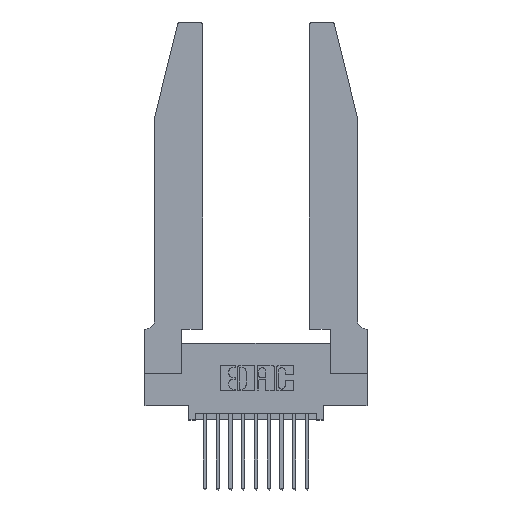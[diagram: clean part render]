
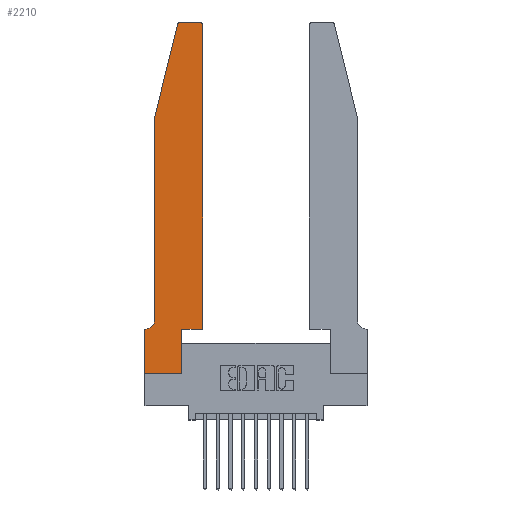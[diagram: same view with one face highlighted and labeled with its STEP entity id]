
A CAD part, top view. The second image highlights one B-rep face of the part: STEP entity #2210.
In plain terms, the highlighted planar face has unit normal (0, 0, 1).
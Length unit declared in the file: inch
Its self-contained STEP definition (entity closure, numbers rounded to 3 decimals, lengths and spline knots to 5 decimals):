
#287 = VERTEX_POINT ( 'NONE', #12899 ) ;
#303 = CARTESIAN_POINT ( 'NONE',  ( 0., 0.35, 0.37 ) ) ;
#448 = CARTESIAN_POINT ( 'NONE',  ( 0.2605, 2.75, 0.37 ) ) ;
#596 = EDGE_CURVE ( 'NONE', #287, #14193, #16428, .T. ) ;
#604 = LINE ( 'NONE', #13085, #7911 ) ;
#709 = CARTESIAN_POINT ( 'NONE',  ( 0., 0.35, 0.37 ) ) ;
#769 = EDGE_CURVE ( 'NONE', #11326, #11092, #8310, .T. ) ;
#1048 = DIRECTION ( 'NONE',  ( 1., 0., 0. ) ) ;
#1059 = EDGE_CURVE ( 'NONE', #14193, #14011, #7301, .T. ) ;
#1336 = EDGE_CURVE ( 'NONE', #14011, #14027, #604, .T. ) ;
#1745 = ORIENTED_EDGE ( 'NONE', *, *, #1059, .T. ) ;
#2008 = LINE ( 'NONE', #12150, #14645 ) ;
#2168 = ORIENTED_EDGE ( 'NONE', *, *, #7573, .T. ) ;
#2210 = ADVANCED_FACE ( 'NONE', ( #2660 ), #14324, .T. ) ;
#2517 = DIRECTION ( 'NONE',  ( 0., 1., 0. ) ) ;
#2660 = FACE_OUTER_BOUND ( 'NONE', #3579, .T. ) ;
#2661 = DIRECTION ( 'NONE',  ( 0., 1., 0. ) ) ;
#2705 = CARTESIAN_POINT ( 'NONE',  ( 0., 0., 0.37 ) ) ;
#2815 = CARTESIAN_POINT ( 'NONE',  ( 0.284, 2.75, 0.37 ) ) ;
#2979 = ORIENTED_EDGE ( 'NONE', *, *, #12276, .T. ) ;
#3173 = EDGE_CURVE ( 'NONE', #13907, #3581, #12299, .T. ) ;
#3411 = CARTESIAN_POINT ( 'NONE',  ( 0., 0., 0.37 ) ) ;
#3579 = EDGE_LOOP ( 'NONE', ( #14785, #1745, #8572, #2168, #8960, #15566, #5998, #2979, #9732, #13031, #16309, #6804 ) ) ;
#3581 = VERTEX_POINT ( 'NONE', #13322 ) ;
#3969 = VECTOR ( 'NONE', #10959, 39.37008 ) ;
#4088 = DIRECTION ( 'NONE',  ( 1., 0., 0. ) ) ;
#4213 = LINE ( 'NONE', #6882, #10891 ) ;
#4274 = EDGE_CURVE ( 'NONE', #3581, #4727, #2008, .T. ) ;
#4333 = VERTEX_POINT ( 'NONE', #6031 ) ;
#4417 = LINE ( 'NONE', #11414, #7799 ) ;
#4620 = VERTEX_POINT ( 'NONE', #2705 ) ;
#4727 = VERTEX_POINT ( 'NONE', #303 ) ;
#5680 = VECTOR ( 'NONE', #11058, 39.37008 ) ;
#5998 = ORIENTED_EDGE ( 'NONE', *, *, #15206, .T. ) ;
#6031 = CARTESIAN_POINT ( 'NONE',  ( 0.2865, 0., 0.37 ) ) ;
#6441 = DIRECTION ( 'NONE',  ( -1., 0., 0. ) ) ;
#6758 = CARTESIAN_POINT ( 'NONE',  ( 0.2865, 0.35, 0.37 ) ) ;
#6804 = ORIENTED_EDGE ( 'NONE', *, *, #9754, .T. ) ;
#6882 = CARTESIAN_POINT ( 'NONE',  ( 0., 0., 0.37 ) ) ;
#7301 = CIRCLE ( 'NONE', #7416, 0.03 ) ;
#7314 = DIRECTION ( 'NONE',  ( 0., 0., 1. ) ) ;
#7416 = AXIS2_PLACEMENT_3D ( 'NONE', #11937, #15334, #4088 ) ;
#7573 = EDGE_CURVE ( 'NONE', #14027, #13907, #9047, .T. ) ;
#7584 = CARTESIAN_POINT ( 'NONE',  ( 0.25487, 2.72718, 0.37 ) ) ;
#7799 = VECTOR ( 'NONE', #2517, 39.37008 ) ;
#7911 = VECTOR ( 'NONE', #13626, 39.37008 ) ;
#7922 = CARTESIAN_POINT ( 'NONE',  ( 0.0055, 0.42, 0.37 ) ) ;
#8040 = LINE ( 'NONE', #8762, #8422 ) ;
#8310 = LINE ( 'NONE', #13267, #11203 ) ;
#8422 = VECTOR ( 'NONE', #1048, 39.37008 ) ;
#8572 = ORIENTED_EDGE ( 'NONE', *, *, #1336, .T. ) ;
#8584 = CARTESIAN_POINT ( 'NONE',  ( 0.0755, 2., 0.37 ) ) ;
#8762 = CARTESIAN_POINT ( 'NONE',  ( 0.4505, 0.35, 0.37 ) ) ;
#8833 = EDGE_CURVE ( 'NONE', #10150, #11326, #8040, .T. ) ;
#8960 = ORIENTED_EDGE ( 'NONE', *, *, #3173, .T. ) ;
#9047 = LINE ( 'NONE', #8584, #5680 ) ;
#9297 = DIRECTION ( 'NONE',  ( 0., 0., 1. ) ) ;
#9319 = DIRECTION ( 'NONE',  ( -1., 0., 0. ) ) ;
#9732 = ORIENTED_EDGE ( 'NONE', *, *, #14957, .T. ) ;
#9754 = EDGE_CURVE ( 'NONE', #11092, #287, #12069, .T. ) ;
#10150 = VERTEX_POINT ( 'NONE', #6758 ) ;
#10278 = LINE ( 'NONE', #3411, #3969 ) ;
#10891 = VECTOR ( 'NONE', #15600, 39.37008 ) ;
#10959 = DIRECTION ( 'NONE',  ( 1., 0., 0. ) ) ;
#11058 = DIRECTION ( 'NONE',  ( 0., -1., 0. ) ) ;
#11092 = VERTEX_POINT ( 'NONE', #11141 ) ;
#11141 = CARTESIAN_POINT ( 'NONE',  ( 0.4505, 2.72, 0.37 ) ) ;
#11203 = VECTOR ( 'NONE', #2661, 39.37008 ) ;
#11324 = CARTESIAN_POINT ( 'NONE',  ( 0.0755, 2., 0.37 ) ) ;
#11326 = VERTEX_POINT ( 'NONE', #12886 ) ;
#11414 = CARTESIAN_POINT ( 'NONE',  ( 0.2865, 0.35, 0.37 ) ) ;
#11937 = CARTESIAN_POINT ( 'NONE',  ( 0.284, 2.72, 0.37 ) ) ;
#12069 = CIRCLE ( 'NONE', #12974, 0.03 ) ;
#12150 = CARTESIAN_POINT ( 'NONE',  ( 0.0755, 0.35, 0.37 ) ) ;
#12276 = EDGE_CURVE ( 'NONE', #4620, #4333, #10278, .T. ) ;
#12299 = CIRCLE ( 'NONE', #16366, 0.07 ) ;
#12886 = CARTESIAN_POINT ( 'NONE',  ( 0.4505, 0.35, 0.37 ) ) ;
#12899 = CARTESIAN_POINT ( 'NONE',  ( 0.4205, 2.75, 0.37 ) ) ;
#12974 = AXIS2_PLACEMENT_3D ( 'NONE', #14779, #7314, #16011 ) ;
#13031 = ORIENTED_EDGE ( 'NONE', *, *, #8833, .T. ) ;
#13085 = CARTESIAN_POINT ( 'NONE',  ( 0.0755, 2., 0.37 ) ) ;
#13155 = VECTOR ( 'NONE', #6441, 39.37008 ) ;
#13157 = AXIS2_PLACEMENT_3D ( 'NONE', #709, #9297, #14214 ) ;
#13267 = CARTESIAN_POINT ( 'NONE',  ( 0.4505, 0.35, 0.37 ) ) ;
#13322 = CARTESIAN_POINT ( 'NONE',  ( 0.0055, 0.35, 0.37 ) ) ;
#13406 = CARTESIAN_POINT ( 'NONE',  ( 0.0755, 0.42, 0.37 ) ) ;
#13413 = DIRECTION ( 'NONE',  ( -1., 0., 0. ) ) ;
#13626 = DIRECTION ( 'NONE',  ( -0.239, -0.971, 0. ) ) ;
#13907 = VERTEX_POINT ( 'NONE', #13406 ) ;
#14011 = VERTEX_POINT ( 'NONE', #7584 ) ;
#14027 = VERTEX_POINT ( 'NONE', #11324 ) ;
#14193 = VERTEX_POINT ( 'NONE', #2815 ) ;
#14214 = DIRECTION ( 'NONE',  ( 1., 0., 0. ) ) ;
#14324 = PLANE ( 'NONE',  #13157 ) ;
#14444 = DIRECTION ( 'NONE',  ( 0., 0., -1. ) ) ;
#14645 = VECTOR ( 'NONE', #13413, 39.37008 ) ;
#14779 = CARTESIAN_POINT ( 'NONE',  ( 0.4205, 2.72, 0.37 ) ) ;
#14785 = ORIENTED_EDGE ( 'NONE', *, *, #596, .T. ) ;
#14957 = EDGE_CURVE ( 'NONE', #4333, #10150, #4417, .T. ) ;
#15206 = EDGE_CURVE ( 'NONE', #4727, #4620, #4213, .T. ) ;
#15334 = DIRECTION ( 'NONE',  ( 0., 0., 1. ) ) ;
#15566 = ORIENTED_EDGE ( 'NONE', *, *, #4274, .T. ) ;
#15600 = DIRECTION ( 'NONE',  ( 0., -1., 0. ) ) ;
#16011 = DIRECTION ( 'NONE',  ( 1., 0., 0. ) ) ;
#16309 = ORIENTED_EDGE ( 'NONE', *, *, #769, .T. ) ;
#16366 = AXIS2_PLACEMENT_3D ( 'NONE', #7922, #14444, #9319 ) ;
#16428 = LINE ( 'NONE', #448, #13155 ) ;
